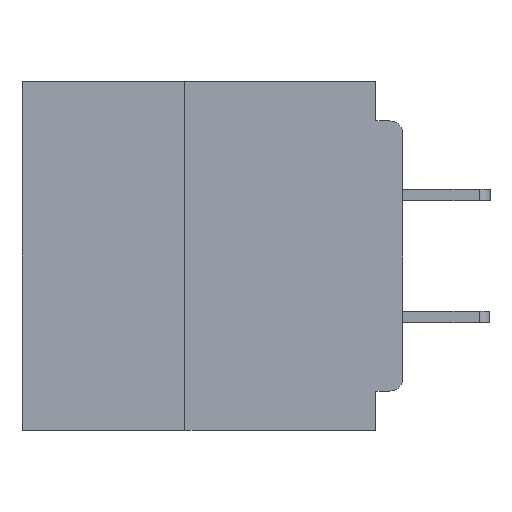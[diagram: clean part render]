
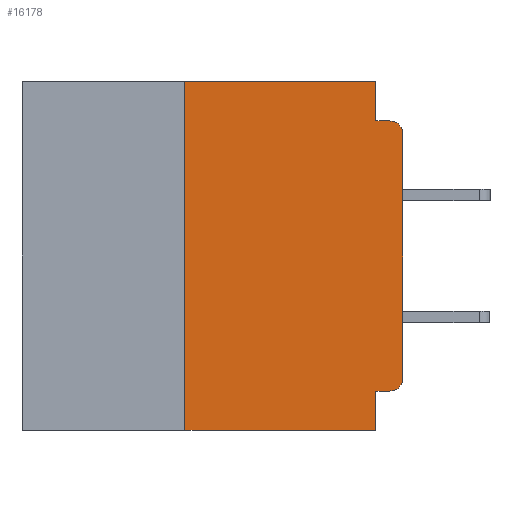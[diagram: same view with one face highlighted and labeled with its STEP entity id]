
A CAD part, left-side view. The second image highlights one B-rep face of the part: STEP entity #16178.
In plain terms, the highlighted planar face has unit normal (-1, 0, 0).
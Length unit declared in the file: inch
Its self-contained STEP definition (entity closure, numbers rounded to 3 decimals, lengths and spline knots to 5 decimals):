
#521 = CARTESIAN_POINT ( 'NONE',  ( 0., 0.031, 0. ) ) ;
#579 = CARTESIAN_POINT ( 'NONE',  ( 0., 0.031, 0. ) ) ;
#1953 = VERTEX_POINT ( 'NONE', #32762 ) ;
#2064 = VERTEX_POINT ( 'NONE', #19863 ) ;
#2355 = DIRECTION ( 'NONE',  ( 0., 0., -1. ) ) ;
#2474 = LINE ( 'NONE', #17433, #11466 ) ;
#2588 = DIRECTION ( 'NONE',  ( 0., 0., 1. ) ) ;
#2708 = LINE ( 'NONE', #26657, #3761 ) ;
#3155 = VERTEX_POINT ( 'NONE', #36518 ) ;
#3761 = VECTOR ( 'NONE', #6568, 39.37008 ) ;
#4271 = DIRECTION ( 'NONE',  ( 0., 0., 1. ) ) ;
#5269 = VECTOR ( 'NONE', #4271, 39.37008 ) ;
#5460 = DIRECTION ( 'NONE',  ( -1., 0., 0. ) ) ;
#6102 = ORIENTED_EDGE ( 'NONE', *, *, #14270, .T. ) ;
#6380 = CIRCLE ( 'NONE', #38019, 0.015 ) ;
#6568 = DIRECTION ( 'NONE',  ( 0., -1., 0. ) ) ;
#6658 = VERTEX_POINT ( 'NONE', #33787 ) ;
#7683 = VECTOR ( 'NONE', #32736, 39.37008 ) ;
#7709 = EDGE_CURVE ( 'NONE', #1953, #24150, #19976, .T. ) ;
#9688 = VERTEX_POINT ( 'NONE', #18342 ) ;
#9876 = CARTESIAN_POINT ( 'NONE',  ( 0., 0.015, -0.045 ) ) ;
#9898 = ORIENTED_EDGE ( 'NONE', *, *, #15556, .F. ) ;
#10107 = VERTEX_POINT ( 'NONE', #579 ) ;
#10597 = CARTESIAN_POINT ( 'NONE',  ( 0., 0.031, -0.045 ) ) ;
#10775 = CARTESIAN_POINT ( 'NONE',  ( 0., 0.437, 0. ) ) ;
#11466 = VECTOR ( 'NONE', #37492, 39.37008 ) ;
#11908 = ORIENTED_EDGE ( 'NONE', *, *, #40283, .F. ) ;
#12869 = AXIS2_PLACEMENT_3D ( 'NONE', #42471, #22455, #2355 ) ;
#13767 = ORIENTED_EDGE ( 'NONE', *, *, #42977, .F. ) ;
#14126 = DIRECTION ( 'NONE',  ( 0., 0., -1. ) ) ;
#14270 = EDGE_CURVE ( 'NONE', #43209, #2064, #2708, .T. ) ;
#14711 = VECTOR ( 'NONE', #27361, 39.37008 ) ;
#15556 = EDGE_CURVE ( 'NONE', #10107, #21516, #24675, .T. ) ;
#15995 = CARTESIAN_POINT ( 'NONE',  ( 0., 0., -0.355 ) ) ;
#16106 = ORIENTED_EDGE ( 'NONE', *, *, #39840, .T. ) ;
#16178 = ADVANCED_FACE ( 'NONE', ( #23021 ), #27451, .F. ) ;
#16231 = DIRECTION ( 'NONE',  ( 0., 0., -1. ) ) ;
#16582 = LINE ( 'NONE', #32782, #24469 ) ;
#17433 = CARTESIAN_POINT ( 'NONE',  ( 0., 0.437, 0. ) ) ;
#17685 = EDGE_CURVE ( 'NONE', #6658, #9688, #16582, .T. ) ;
#18342 = CARTESIAN_POINT ( 'NONE',  ( 0., 0., -0.06 ) ) ;
#18360 = EDGE_CURVE ( 'NONE', #21516, #28631, #24930, .T. ) ;
#18461 = ORIENTED_EDGE ( 'NONE', *, *, #28500, .T. ) ;
#18996 = ORIENTED_EDGE ( 'NONE', *, *, #7709, .F. ) ;
#19863 = CARTESIAN_POINT ( 'NONE',  ( 0., 0.031, -0.4 ) ) ;
#19976 = LINE ( 'NONE', #15995, #27875 ) ;
#21516 = VERTEX_POINT ( 'NONE', #10597 ) ;
#22455 = DIRECTION ( 'NONE',  ( -1., 0., 0. ) ) ;
#23021 = FACE_OUTER_BOUND ( 'NONE', #23748, .T. ) ;
#23467 = CARTESIAN_POINT ( 'NONE',  ( 0., 0.031, -0.355 ) ) ;
#23748 = EDGE_LOOP ( 'NONE', ( #28793, #16106, #38985, #9898, #13767, #11908, #6102, #40969, #18996, #18461 ) ) ;
#24150 = VERTEX_POINT ( 'NONE', #23467 ) ;
#24469 = VECTOR ( 'NONE', #2588, 39.37008 ) ;
#24675 = LINE ( 'NONE', #521, #14711 ) ;
#24930 = LINE ( 'NONE', #36105, #7683 ) ;
#25594 = CARTESIAN_POINT ( 'NONE',  ( 0., 0.015, -0.06 ) ) ;
#26657 = CARTESIAN_POINT ( 'NONE',  ( 0., 0.437, -0.4 ) ) ;
#27085 = CIRCLE ( 'NONE', #12869, 0.015 ) ;
#27361 = DIRECTION ( 'NONE',  ( 0., 0., -1. ) ) ;
#27451 = PLANE ( 'NONE',  #33852 ) ;
#27875 = VECTOR ( 'NONE', #42752, 39.37008 ) ;
#28500 = EDGE_CURVE ( 'NONE', #1953, #6658, #27085, .T. ) ;
#28631 = VERTEX_POINT ( 'NONE', #9876 ) ;
#28698 = CARTESIAN_POINT ( 'NONE',  ( 0., 0.25, -0.4 ) ) ;
#28793 = ORIENTED_EDGE ( 'NONE', *, *, #17685, .T. ) ;
#28931 = DIRECTION ( 'NONE',  ( 0., 0., -1. ) ) ;
#29193 = EDGE_CURVE ( 'NONE', #24150, #2064, #33276, .T. ) ;
#31085 = CARTESIAN_POINT ( 'NONE',  ( 0., 0.25, -0.4 ) ) ;
#32736 = DIRECTION ( 'NONE',  ( 0., -1., 0. ) ) ;
#32762 = CARTESIAN_POINT ( 'NONE',  ( 0., 0.015, -0.355 ) ) ;
#32782 = CARTESIAN_POINT ( 'NONE',  ( 0., 0., 0. ) ) ;
#33276 = LINE ( 'NONE', #36291, #43201 ) ;
#33787 = CARTESIAN_POINT ( 'NONE',  ( 0., 0., -0.34 ) ) ;
#33852 = AXIS2_PLACEMENT_3D ( 'NONE', #10775, #34173, #14126 ) ;
#34173 = DIRECTION ( 'NONE',  ( 1., 0., 0. ) ) ;
#36105 = CARTESIAN_POINT ( 'NONE',  ( 0., 0., -0.045 ) ) ;
#36291 = CARTESIAN_POINT ( 'NONE',  ( 0., 0.031, -0.4 ) ) ;
#36518 = CARTESIAN_POINT ( 'NONE',  ( 0., 0.25, 0. ) ) ;
#37492 = DIRECTION ( 'NONE',  ( 0., -1., 0. ) ) ;
#38019 = AXIS2_PLACEMENT_3D ( 'NONE', #25594, #5460, #28931 ) ;
#38843 = LINE ( 'NONE', #31085, #5269 ) ;
#38985 = ORIENTED_EDGE ( 'NONE', *, *, #18360, .F. ) ;
#39840 = EDGE_CURVE ( 'NONE', #9688, #28631, #6380, .T. ) ;
#40283 = EDGE_CURVE ( 'NONE', #43209, #3155, #38843, .T. ) ;
#40969 = ORIENTED_EDGE ( 'NONE', *, *, #29193, .F. ) ;
#42471 = CARTESIAN_POINT ( 'NONE',  ( 0., 0.015, -0.34 ) ) ;
#42752 = DIRECTION ( 'NONE',  ( 0., 1., 0. ) ) ;
#42977 = EDGE_CURVE ( 'NONE', #3155, #10107, #2474, .T. ) ;
#43201 = VECTOR ( 'NONE', #16231, 39.37008 ) ;
#43209 = VERTEX_POINT ( 'NONE', #28698 ) ;
